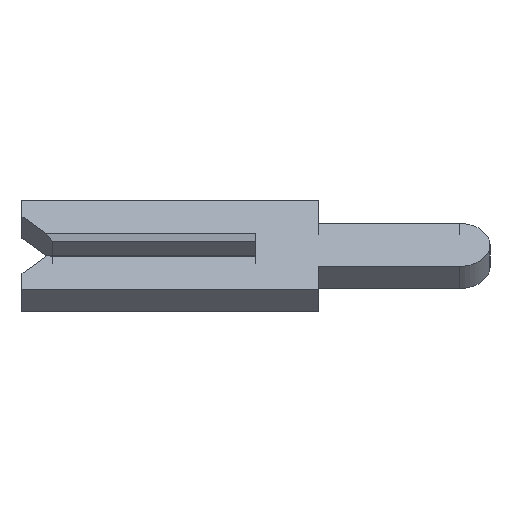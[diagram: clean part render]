
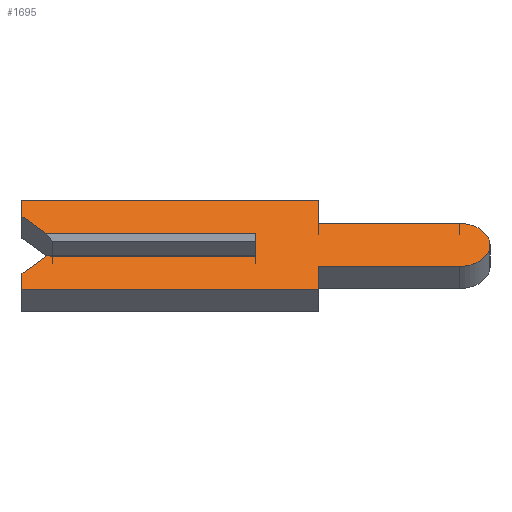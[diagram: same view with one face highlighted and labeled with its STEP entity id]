
A CAD part, left-side view. The second image highlights one B-rep face of the part: STEP entity #1695.
In plain terms, the highlighted face is planar.
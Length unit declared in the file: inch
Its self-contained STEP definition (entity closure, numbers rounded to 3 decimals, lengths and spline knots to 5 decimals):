
#3 = ORIENTED_EDGE ( 'NONE', *, *, #1983, .F. ) ;
#9 = DIRECTION ( 'NONE',  ( 0., 1., 0. ) ) ;
#16 = DIRECTION ( 'NONE',  ( 0., -1., 0. ) ) ;
#50 = DIRECTION ( 'NONE',  ( 0., 0., -1. ) ) ;
#77 = CARTESIAN_POINT ( 'NONE',  ( -0.01, 0.15, 0.01 ) ) ;
#107 = EDGE_LOOP ( 'NONE', ( #998, #1741, #2005, #1362, #1445, #1153, #1788, #517, #1085, #157, #1650, #1747, #1231, #3 ) ) ;
#137 = FACE_OUTER_BOUND ( 'NONE', #107, .T. ) ;
#142 = EDGE_CURVE ( 'NONE', #330, #1768, #1675, .T. ) ;
#157 = ORIENTED_EDGE ( 'NONE', *, *, #1997, .F. ) ;
#161 = LINE ( 'NONE', #1759, #936 ) ;
#171 = CARTESIAN_POINT ( 'NONE',  ( -0.01, -0.1305, 0. ) ) ;
#193 = DIRECTION ( 'NONE',  ( 0., 0.707, 0.707 ) ) ;
#226 = VERTEX_POINT ( 'NONE', #683 ) ;
#233 = DIRECTION ( 'NONE',  ( 0., -1., 0. ) ) ;
#242 = VECTOR ( 'NONE', #1263, 39.37008 ) ;
#295 = CARTESIAN_POINT ( 'NONE',  ( -0.01, -0.04, -0.0195 ) ) ;
#330 = VERTEX_POINT ( 'NONE', #1174 ) ;
#340 = CARTESIAN_POINT ( 'NONE',  ( -0.01, 0.1305, 0.0065 ) ) ;
#343 = VECTOR ( 'NONE', #1587, 39.37008 ) ;
#360 = EDGE_CURVE ( 'NONE', #1386, #1376, #1098, .T. ) ;
#371 = CARTESIAN_POINT ( 'NONE',  ( -0.01, 0.15, 0.04 ) ) ;
#375 = CIRCLE ( 'NONE', #417, 0.0195 ) ;
#389 = AXIS2_PLACEMENT_3D ( 'NONE', #171, #1119, #653 ) ;
#417 = AXIS2_PLACEMENT_3D ( 'NONE', #1639, #1478, #1322 ) ;
#434 = CARTESIAN_POINT ( 'NONE',  ( -0.01, 0.15, 0.04 ) ) ;
#462 = LINE ( 'NONE', #77, #1126 ) ;
#469 = CARTESIAN_POINT ( 'NONE',  ( -0.01, 0.134, -0.01 ) ) ;
#479 = EDGE_CURVE ( 'NONE', #1591, #1913, #375, .T. ) ;
#480 = CARTESIAN_POINT ( 'NONE',  ( -0.01, -0.04, -0.04 ) ) ;
#492 = CARTESIAN_POINT ( 'NONE',  ( -0.01, -0.1305, 0.0195 ) ) ;
#517 = ORIENTED_EDGE ( 'NONE', *, *, #1146, .F. ) ;
#518 = EDGE_CURVE ( 'NONE', #1376, #1872, #1148, .T. ) ;
#544 = LINE ( 'NONE', #480, #1061 ) ;
#600 = EDGE_CURVE ( 'NONE', #1466, #1423, #462, .T. ) ;
#619 = CARTESIAN_POINT ( 'NONE',  ( -0.01, -0.1305, -0.01 ) ) ;
#653 = DIRECTION ( 'NONE',  ( 0., 0., -1. ) ) ;
#683 = CARTESIAN_POINT ( 'NONE',  ( -0.01, -0.04, -0.04 ) ) ;
#765 = DIRECTION ( 'NONE',  ( 0., 1., 0. ) ) ;
#776 = VECTOR ( 'NONE', #193, 39.37008 ) ;
#805 = CARTESIAN_POINT ( 'NONE',  ( -0.01, 0.15, -0.04 ) ) ;
#830 = CARTESIAN_POINT ( 'NONE',  ( -0.01, -0.1305, -0.0195 ) ) ;
#846 = VECTOR ( 'NONE', #765, 39.37008 ) ;
#909 = CARTESIAN_POINT ( 'NONE',  ( -0.01, -0.04, -0.0195 ) ) ;
#936 = VECTOR ( 'NONE', #1446, 39.37008 ) ;
#981 = LINE ( 'NONE', #619, #242 ) ;
#984 = CARTESIAN_POINT ( 'NONE',  ( -0.01, -0.04, 0.04 ) ) ;
#998 = ORIENTED_EDGE ( 'NONE', *, *, #600, .T. ) ;
#1001 = DIRECTION ( 'NONE',  ( 0., -1., 0. ) ) ;
#1009 = LINE ( 'NONE', #295, #846 ) ;
#1033 = LINE ( 'NONE', #805, #1091 ) ;
#1061 = VECTOR ( 'NONE', #50, 39.37008 ) ;
#1063 = CARTESIAN_POINT ( 'NONE',  ( -0.01, 0.15, 0.026 ) ) ;
#1085 = ORIENTED_EDGE ( 'NONE', *, *, #479, .F. ) ;
#1086 = CARTESIAN_POINT ( 'NONE',  ( -0.01, 0.15, -0.026 ) ) ;
#1091 = VECTOR ( 'NONE', #9, 39.37008 ) ;
#1098 = LINE ( 'NONE', #1656, #1860 ) ;
#1107 = VECTOR ( 'NONE', #16, 39.37008 ) ;
#1119 = DIRECTION ( 'NONE',  ( 1., 0., 0. ) ) ;
#1126 = VECTOR ( 'NONE', #233, 39.37008 ) ;
#1146 = EDGE_CURVE ( 'NONE', #1913, #1201, #1009, .T. ) ;
#1148 = LINE ( 'NONE', #371, #1458 ) ;
#1153 = ORIENTED_EDGE ( 'NONE', *, *, #1524, .F. ) ;
#1174 = CARTESIAN_POINT ( 'NONE',  ( -0.01, 0.15, -0.026 ) ) ;
#1201 = VERTEX_POINT ( 'NONE', #909 ) ;
#1231 = ORIENTED_EDGE ( 'NONE', *, *, #360, .F. ) ;
#1255 = LINE ( 'NONE', #1269, #343 ) ;
#1259 = VECTOR ( 'NONE', #1538, 39.37008 ) ;
#1260 = CARTESIAN_POINT ( 'NONE',  ( -0.01, 0., 0.01 ) ) ;
#1263 = DIRECTION ( 'NONE',  ( 0., -1., 0. ) ) ;
#1269 = CARTESIAN_POINT ( 'NONE',  ( -0.01, -0.04, 0.04 ) ) ;
#1302 = CARTESIAN_POINT ( 'NONE',  ( -0.01, 0.1305, -0.0065 ) ) ;
#1322 = DIRECTION ( 'NONE',  ( 0., 0., -1. ) ) ;
#1336 = EDGE_CURVE ( 'NONE', #1920, #330, #1690, .T. ) ;
#1341 = VERTEX_POINT ( 'NONE', #2006 ) ;
#1362 = ORIENTED_EDGE ( 'NONE', *, *, #142, .F. ) ;
#1376 = VERTEX_POINT ( 'NONE', #434 ) ;
#1386 = VERTEX_POINT ( 'NONE', #1063 ) ;
#1397 = PLANE ( 'NONE',  #389 ) ;
#1423 = VERTEX_POINT ( 'NONE', #1260 ) ;
#1440 = EDGE_CURVE ( 'NONE', #1872, #1341, #1255, .T. ) ;
#1445 = ORIENTED_EDGE ( 'NONE', *, *, #1336, .F. ) ;
#1446 = DIRECTION ( 'NONE',  ( 0., 0., 1. ) ) ;
#1458 = VECTOR ( 'NONE', #1001, 39.37008 ) ;
#1459 = VECTOR ( 'NONE', #1592, 39.37008 ) ;
#1466 = VERTEX_POINT ( 'NONE', #1582 ) ;
#1469 = VERTEX_POINT ( 'NONE', #1896 ) ;
#1478 = DIRECTION ( 'NONE',  ( 1., 0., 0. ) ) ;
#1524 = EDGE_CURVE ( 'NONE', #226, #1920, #1033, .T. ) ;
#1538 = DIRECTION ( 'NONE',  ( 0., 0., 1. ) ) ;
#1582 = CARTESIAN_POINT ( 'NONE',  ( -0.01, 0.134, 0.01 ) ) ;
#1587 = DIRECTION ( 'NONE',  ( 0., 0., -1. ) ) ;
#1591 = VERTEX_POINT ( 'NONE', #492 ) ;
#1592 = DIRECTION ( 'NONE',  ( 0., -0.707, 0.707 ) ) ;
#1621 = LINE ( 'NONE', #340, #776 ) ;
#1624 = CARTESIAN_POINT ( 'NONE',  ( -0.01, -0.04, 0.0195 ) ) ;
#1639 = CARTESIAN_POINT ( 'NONE',  ( -0.01, -0.1305, 0. ) ) ;
#1650 = ORIENTED_EDGE ( 'NONE', *, *, #1440, .F. ) ;
#1656 = CARTESIAN_POINT ( 'NONE',  ( -0.01, 0.15, 0.026 ) ) ;
#1675 = LINE ( 'NONE', #1302, #1459 ) ;
#1683 = EDGE_CURVE ( 'NONE', #1768, #1469, #981, .T. ) ;
#1690 = LINE ( 'NONE', #1086, #1259 ) ;
#1695 = ADVANCED_FACE ( 'NONE', ( #137 ), #1397, .F. ) ;
#1741 = ORIENTED_EDGE ( 'NONE', *, *, #1820, .F. ) ;
#1747 = ORIENTED_EDGE ( 'NONE', *, *, #518, .F. ) ;
#1759 = CARTESIAN_POINT ( 'NONE',  ( -0.01, 0., 0.0065 ) ) ;
#1768 = VERTEX_POINT ( 'NONE', #469 ) ;
#1784 = EDGE_CURVE ( 'NONE', #1201, #226, #544, .T. ) ;
#1788 = ORIENTED_EDGE ( 'NONE', *, *, #1784, .F. ) ;
#1820 = EDGE_CURVE ( 'NONE', #1469, #1423, #161, .T. ) ;
#1860 = VECTOR ( 'NONE', #1931, 39.37008 ) ;
#1872 = VERTEX_POINT ( 'NONE', #984 ) ;
#1896 = CARTESIAN_POINT ( 'NONE',  ( -0.01, 0., -0.01 ) ) ;
#1913 = VERTEX_POINT ( 'NONE', #830 ) ;
#1920 = VERTEX_POINT ( 'NONE', #1929 ) ;
#1929 = CARTESIAN_POINT ( 'NONE',  ( -0.01, 0.15, -0.04 ) ) ;
#1930 = LINE ( 'NONE', #1624, #1107 ) ;
#1931 = DIRECTION ( 'NONE',  ( 0., 0., 1. ) ) ;
#1983 = EDGE_CURVE ( 'NONE', #1466, #1386, #1621, .T. ) ;
#1997 = EDGE_CURVE ( 'NONE', #1341, #1591, #1930, .T. ) ;
#2005 = ORIENTED_EDGE ( 'NONE', *, *, #1683, .F. ) ;
#2006 = CARTESIAN_POINT ( 'NONE',  ( -0.01, -0.04, 0.0195 ) ) ;
